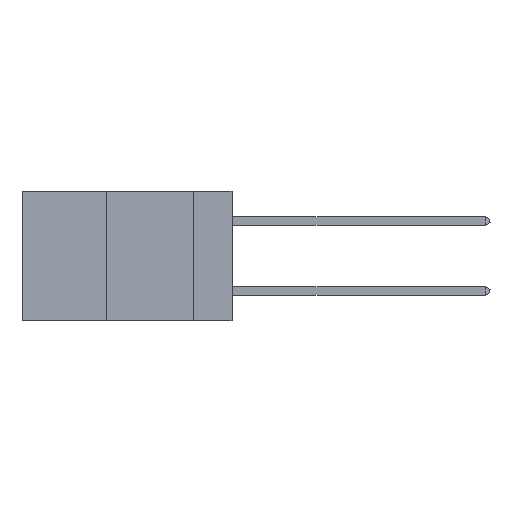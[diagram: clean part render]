
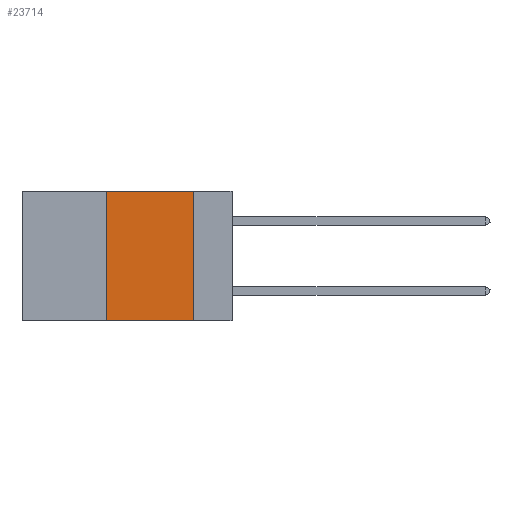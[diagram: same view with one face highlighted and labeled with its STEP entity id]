
A CAD part, left-side view. The second image highlights one B-rep face of the part: STEP entity #23714.
In plain terms, the highlighted planar face has unit normal (-1, 0, 0).
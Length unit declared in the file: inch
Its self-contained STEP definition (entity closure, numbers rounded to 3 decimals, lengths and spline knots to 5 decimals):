
#39 = DIRECTION ( 'NONE',  ( 0., -1., 0. ) ) ;
#331 = LINE ( 'NONE', #15721, #6915 ) ;
#1409 = VERTEX_POINT ( 'NONE', #14190 ) ;
#1536 = CARTESIAN_POINT ( 'NONE',  ( 0., 0.36, -0.37 ) ) ;
#1562 = EDGE_CURVE ( 'NONE', #6241, #1409, #2863, .T. ) ;
#2374 = LINE ( 'NONE', #10024, #14898 ) ;
#2863 = LINE ( 'NONE', #25812, #14389 ) ;
#2968 = EDGE_CURVE ( 'NONE', #1409, #14681, #15558, .T. ) ;
#4001 = DIRECTION ( 'NONE',  ( 0., 0., -1. ) ) ;
#4131 = AXIS2_PLACEMENT_3D ( 'NONE', #10909, #22966, #8660 ) ;
#4310 = VECTOR ( 'NONE', #11928, 39.37008 ) ;
#6241 = VERTEX_POINT ( 'NONE', #1536 ) ;
#6520 = CARTESIAN_POINT ( 'NONE',  ( 0., 0.11, -0.37 ) ) ;
#6733 = PLANE ( 'NONE',  #4131 ) ;
#6915 = VECTOR ( 'NONE', #39, 39.37008 ) ;
#7211 = EDGE_LOOP ( 'NONE', ( #16540, #23321, #15487, #15463 ) ) ;
#8519 = VERTEX_POINT ( 'NONE', #6520 ) ;
#8660 = DIRECTION ( 'NONE',  ( 0., 0., -1. ) ) ;
#10024 = CARTESIAN_POINT ( 'NONE',  ( 0., 0.11, 0. ) ) ;
#10909 = CARTESIAN_POINT ( 'NONE',  ( 0., 0.6, 0. ) ) ;
#11928 = DIRECTION ( 'NONE',  ( 0., -1., 0. ) ) ;
#12383 = FACE_OUTER_BOUND ( 'NONE', #7211, .T. ) ;
#13238 = CARTESIAN_POINT ( 'NONE',  ( 0., 0.11, 0. ) ) ;
#14190 = CARTESIAN_POINT ( 'NONE',  ( 0., 0.36, 0. ) ) ;
#14389 = VECTOR ( 'NONE', #15834, 39.37008 ) ;
#14681 = VERTEX_POINT ( 'NONE', #13238 ) ;
#14898 = VECTOR ( 'NONE', #4001, 39.37008 ) ;
#15463 = ORIENTED_EDGE ( 'NONE', *, *, #16831, .T. ) ;
#15487 = ORIENTED_EDGE ( 'NONE', *, *, #1562, .F. ) ;
#15558 = LINE ( 'NONE', #17828, #4310 ) ;
#15721 = CARTESIAN_POINT ( 'NONE',  ( 0., 0.6, -0.37 ) ) ;
#15834 = DIRECTION ( 'NONE',  ( 0., 0., 1. ) ) ;
#16540 = ORIENTED_EDGE ( 'NONE', *, *, #24017, .F. ) ;
#16831 = EDGE_CURVE ( 'NONE', #6241, #8519, #331, .T. ) ;
#17828 = CARTESIAN_POINT ( 'NONE',  ( 0., 0.6, 0. ) ) ;
#22966 = DIRECTION ( 'NONE',  ( 1., 0., 0. ) ) ;
#23321 = ORIENTED_EDGE ( 'NONE', *, *, #2968, .F. ) ;
#23714 = ADVANCED_FACE ( 'NONE', ( #12383 ), #6733, .F. ) ;
#24017 = EDGE_CURVE ( 'NONE', #14681, #8519, #2374, .T. ) ;
#25812 = CARTESIAN_POINT ( 'NONE',  ( 0., 0.36, 0. ) ) ;
